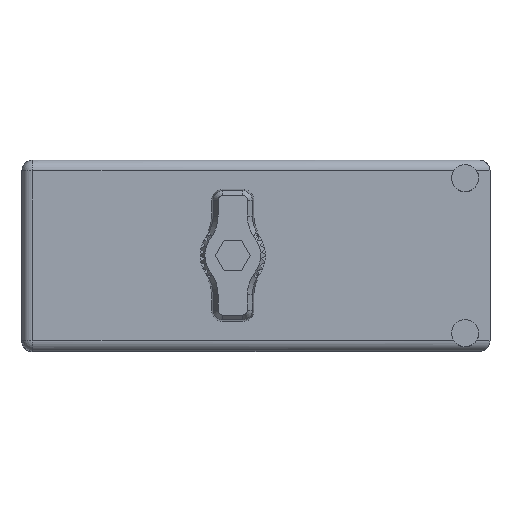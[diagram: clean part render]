
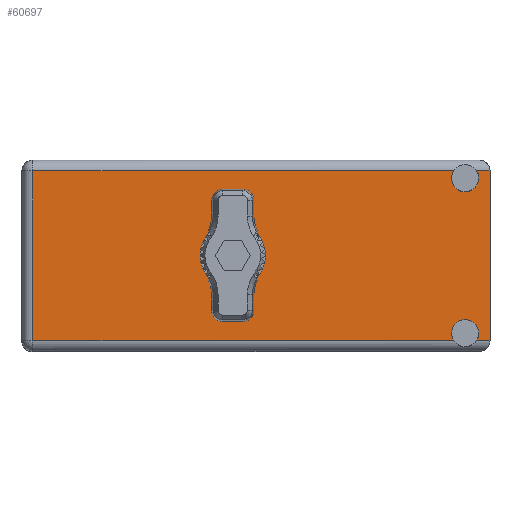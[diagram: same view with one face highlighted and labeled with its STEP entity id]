
A CAD part, top view. The second image highlights one B-rep face of the part: STEP entity #60697.
In plain terms, the highlighted face is planar.
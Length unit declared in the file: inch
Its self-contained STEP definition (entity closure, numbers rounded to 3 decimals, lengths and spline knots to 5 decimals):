
#961 = DIRECTION ( 'NONE',  ( 0., 1., 0. ) ) ;
#2892 = VERTEX_POINT ( 'NONE', #86634 ) ;
#4148 = CIRCLE ( 'NONE', #73111, 0.125 ) ;
#4637 = CARTESIAN_POINT ( 'NONE',  ( 1.359, 1.775, -0.617 ) ) ;
#4866 = CARTESIAN_POINT ( 'NONE',  ( 0., 1.775, -1.164 ) ) ;
#5663 = VECTOR ( 'NONE', #47100, 39.37008 ) ;
#6096 = VERTEX_POINT ( 'NONE', #27995 ) ;
#8967 = LINE ( 'NONE', #62776, #5663 ) ;
#9595 = ORIENTED_EDGE ( 'NONE', *, *, #46145, .F. ) ;
#10465 = CARTESIAN_POINT ( 'NONE',  ( 3.018, 1.775, -0.07 ) ) ;
#11864 = DIRECTION ( 'NONE',  ( 0., 0., 1. ) ) ;
#13552 = DIRECTION ( 'NONE',  ( 0., 1., 0. ) ) ;
#13653 = LINE ( 'NONE', #84996, #82294 ) ;
#14816 = AXIS2_PLACEMENT_3D ( 'NONE', #65195, #961, #29214 ) ;
#15219 = PLANE ( 'NONE',  #41097 ) ;
#16385 = DIRECTION ( 'NONE',  ( 0., 1., 0. ) ) ;
#16752 = EDGE_LOOP ( 'NONE', ( #63050, #50667 ) ) ;
#17452 = CARTESIAN_POINT ( 'NONE',  ( 2.78419, 1.775, -0.07 ) ) ;
#19711 = EDGE_CURVE ( 'NONE', #49502, #83934, #4148, .T. ) ;
#20775 = FACE_OUTER_BOUND ( 'NONE', #74692, .T. ) ;
#23587 = ORIENTED_EDGE ( 'NONE', *, *, #81620, .T. ) ;
#23623 = AXIS2_PLACEMENT_3D ( 'NONE', #86916, #38485, #43874 ) ;
#23640 = LINE ( 'NONE', #54343, #36025 ) ;
#24011 = ORIENTED_EDGE ( 'NONE', *, *, #53024, .F. ) ;
#24023 = CIRCLE ( 'NONE', #75611, 0.0875 ) ;
#24893 = DIRECTION ( 'NONE',  ( 1., 0., 0. ) ) ;
#25630 = DIRECTION ( 'NONE',  ( 1., 0., 0. ) ) ;
#27369 = EDGE_CURVE ( 'NONE', #84422, #85392, #59567, .T. ) ;
#27937 = CARTESIAN_POINT ( 'NONE',  ( 1.359, 1.775, -0.617 ) ) ;
#27995 = CARTESIAN_POINT ( 'NONE',  ( 0.07, 1.775, -0.07 ) ) ;
#28581 = EDGE_CURVE ( 'NONE', #75308, #83156, #83053, .T. ) ;
#29214 = DIRECTION ( 'NONE',  ( 0., 0., 1. ) ) ;
#30360 = CIRCLE ( 'NONE', #23623, 0.0875 ) ;
#31203 = ORIENTED_EDGE ( 'NONE', *, *, #27369, .F. ) ;
#33538 = DIRECTION ( 'NONE',  ( 0., 1., 0. ) ) ;
#33665 = DIRECTION ( 'NONE',  ( 0., 0., 1. ) ) ;
#34149 = CARTESIAN_POINT ( 'NONE',  ( 3.018, 1.775, -1.164 ) ) ;
#34236 = VERTEX_POINT ( 'NONE', #48726 ) ;
#35230 = DIRECTION ( 'NONE',  ( 0., 0., 1. ) ) ;
#36025 = VECTOR ( 'NONE', #25630, 39.37008 ) ;
#38485 = DIRECTION ( 'NONE',  ( 0., 1., 0. ) ) ;
#39761 = CARTESIAN_POINT ( 'NONE',  ( 2.93181, 1.775, -1.164 ) ) ;
#40803 = VERTEX_POINT ( 'NONE', #39761 ) ;
#41097 = AXIS2_PLACEMENT_3D ( 'NONE', #75012, #86934, #88806 ) ;
#43658 = EDGE_CURVE ( 'NONE', #2892, #63078, #24023, .T. ) ;
#43874 = DIRECTION ( 'NONE',  ( 0., 0., 1. ) ) ;
#44361 = LINE ( 'NONE', #10465, #62388 ) ;
#44792 = ORIENTED_EDGE ( 'NONE', *, *, #45992, .T. ) ;
#44879 = CARTESIAN_POINT ( 'NONE',  ( 2.858, 1.775, -0.2045 ) ) ;
#45992 = EDGE_CURVE ( 'NONE', #84422, #40803, #13653, .T. ) ;
#46145 = EDGE_CURVE ( 'NONE', #63078, #40803, #79957, .T. ) ;
#46561 = AXIS2_PLACEMENT_3D ( 'NONE', #56113, #93086, #35230 ) ;
#46781 = FACE_BOUND ( 'NONE', #16752, .T. ) ;
#46894 = CARTESIAN_POINT ( 'NONE',  ( 2.858, 1.775, -1.0295 ) ) ;
#47100 = DIRECTION ( 'NONE',  ( 0., 0., 1. ) ) ;
#48068 = CIRCLE ( 'NONE', #49343, 0.125 ) ;
#48726 = CARTESIAN_POINT ( 'NONE',  ( 2.93181, 1.775, -0.07 ) ) ;
#49343 = AXIS2_PLACEMENT_3D ( 'NONE', #4637, #33538, #11864 ) ;
#49502 = VERTEX_POINT ( 'NONE', #64569 ) ;
#50667 = ORIENTED_EDGE ( 'NONE', *, *, #84397, .F. ) ;
#53024 = EDGE_CURVE ( 'NONE', #34236, #75308, #30360, .T. ) ;
#53476 = ORIENTED_EDGE ( 'NONE', *, *, #28581, .F. ) ;
#54343 = CARTESIAN_POINT ( 'NONE',  ( 3.018, 1.775, -0.07 ) ) ;
#54363 = ORIENTED_EDGE ( 'NONE', *, *, #86047, .T. ) ;
#56113 = CARTESIAN_POINT ( 'NONE',  ( 2.858, 1.775, -0.117 ) ) ;
#58168 = CARTESIAN_POINT ( 'NONE',  ( 0.07, 1.775, -1.164 ) ) ;
#59567 = LINE ( 'NONE', #69346, #76421 ) ;
#60697 = ADVANCED_FACE ( 'NONE', ( #46781, #20775 ), #15219, .T. ) ;
#60793 = CARTESIAN_POINT ( 'NONE',  ( 2.858, 1.775, -1.117 ) ) ;
#60939 = ORIENTED_EDGE ( 'NONE', *, *, #63784, .T. ) ;
#62311 = EDGE_CURVE ( 'NONE', #2892, #81347, #73478, .T. ) ;
#62388 = VECTOR ( 'NONE', #24893, 39.37008 ) ;
#62458 = DIRECTION ( 'NONE',  ( -1., 0., 0. ) ) ;
#62776 = CARTESIAN_POINT ( 'NONE',  ( 0.07, 1.775, -1.234 ) ) ;
#63050 = ORIENTED_EDGE ( 'NONE', *, *, #19711, .F. ) ;
#63078 = VERTEX_POINT ( 'NONE', #46894 ) ;
#63784 = EDGE_CURVE ( 'NONE', #81347, #6096, #8967, .T. ) ;
#64569 = CARTESIAN_POINT ( 'NONE',  ( 1.359, 1.775, -0.492 ) ) ;
#65195 = CARTESIAN_POINT ( 'NONE',  ( 2.858, 1.775, -1.117 ) ) ;
#69346 = CARTESIAN_POINT ( 'NONE',  ( 3.018, 1.775, 0. ) ) ;
#72613 = ORIENTED_EDGE ( 'NONE', *, *, #43658, .F. ) ;
#73111 = AXIS2_PLACEMENT_3D ( 'NONE', #27937, #13552, #92444 ) ;
#73478 = LINE ( 'NONE', #4866, #83525 ) ;
#74692 = EDGE_LOOP ( 'NONE', ( #23587, #53476, #24011, #54363, #31203, #44792, #9595, #72613, #85362, #60939 ) ) ;
#75012 = CARTESIAN_POINT ( 'NONE',  ( 0., 1.775, -1.234 ) ) ;
#75308 = VERTEX_POINT ( 'NONE', #44879 ) ;
#75611 = AXIS2_PLACEMENT_3D ( 'NONE', #60793, #16385, #80877 ) ;
#76421 = VECTOR ( 'NONE', #33665, 39.37008 ) ;
#78394 = DIRECTION ( 'NONE',  ( -1., 0., 0. ) ) ;
#78653 = CARTESIAN_POINT ( 'NONE',  ( 1.359, 1.775, -0.742 ) ) ;
#79957 = CIRCLE ( 'NONE', #14816, 0.0875 ) ;
#80877 = DIRECTION ( 'NONE',  ( 0., 0., 1. ) ) ;
#81347 = VERTEX_POINT ( 'NONE', #58168 ) ;
#81620 = EDGE_CURVE ( 'NONE', #6096, #83156, #23640, .T. ) ;
#81651 = CARTESIAN_POINT ( 'NONE',  ( 3.018, 1.775, -0.07 ) ) ;
#82294 = VECTOR ( 'NONE', #78394, 39.37008 ) ;
#83053 = CIRCLE ( 'NONE', #46561, 0.0875 ) ;
#83156 = VERTEX_POINT ( 'NONE', #17452 ) ;
#83525 = VECTOR ( 'NONE', #62458, 39.37008 ) ;
#83934 = VERTEX_POINT ( 'NONE', #78653 ) ;
#84397 = EDGE_CURVE ( 'NONE', #83934, #49502, #48068, .T. ) ;
#84422 = VERTEX_POINT ( 'NONE', #34149 ) ;
#84996 = CARTESIAN_POINT ( 'NONE',  ( 0., 1.775, -1.164 ) ) ;
#85362 = ORIENTED_EDGE ( 'NONE', *, *, #62311, .T. ) ;
#85392 = VERTEX_POINT ( 'NONE', #81651 ) ;
#86047 = EDGE_CURVE ( 'NONE', #34236, #85392, #44361, .T. ) ;
#86634 = CARTESIAN_POINT ( 'NONE',  ( 2.78419, 1.775, -1.164 ) ) ;
#86916 = CARTESIAN_POINT ( 'NONE',  ( 2.858, 1.775, -0.117 ) ) ;
#86934 = DIRECTION ( 'NONE',  ( 0., 1., 0. ) ) ;
#88806 = DIRECTION ( 'NONE',  ( 0., 0., 1. ) ) ;
#92444 = DIRECTION ( 'NONE',  ( 0., 0., 1. ) ) ;
#93086 = DIRECTION ( 'NONE',  ( 0., 1., 0. ) ) ;
